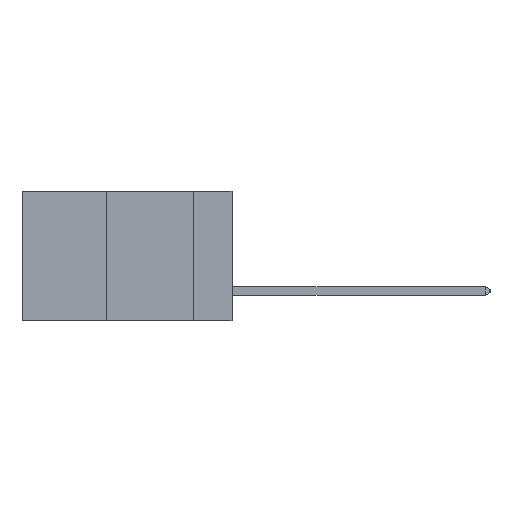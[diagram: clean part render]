
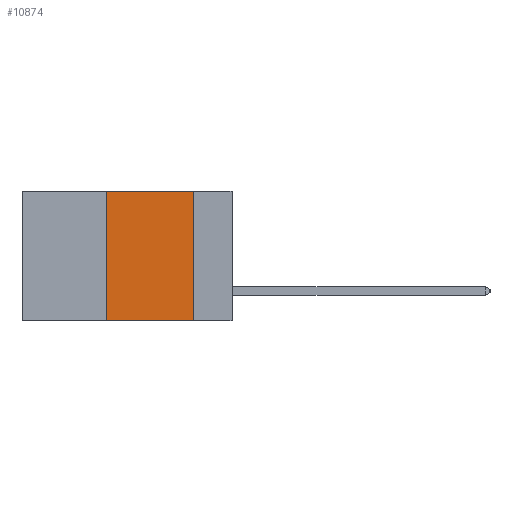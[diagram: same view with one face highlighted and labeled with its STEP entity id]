
A CAD part, left-side view. The second image highlights one B-rep face of the part: STEP entity #10874.
In plain terms, the highlighted planar face has unit normal (-1, 0, 0).
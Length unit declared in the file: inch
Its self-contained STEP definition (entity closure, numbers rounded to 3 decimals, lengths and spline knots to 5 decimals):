
#123 = CARTESIAN_POINT ( 'NONE',  ( 0., 0.6, -0.37 ) ) ;
#626 = ORIENTED_EDGE ( 'NONE', *, *, #4602, .F. ) ;
#1058 = DIRECTION ( 'NONE',  ( 0., 0., -1. ) ) ;
#1191 = AXIS2_PLACEMENT_3D ( 'NONE', #15369, #9246, #1058 ) ;
#1543 = DIRECTION ( 'NONE',  ( 0., -1., 0. ) ) ;
#2613 = CARTESIAN_POINT ( 'NONE',  ( 0., 0.11, 0. ) ) ;
#3537 = DIRECTION ( 'NONE',  ( 0., -1., 0. ) ) ;
#3974 = DIRECTION ( 'NONE',  ( 0., 0., -1. ) ) ;
#4198 = VECTOR ( 'NONE', #1543, 39.37008 ) ;
#4602 = EDGE_CURVE ( 'NONE', #4780, #7732, #5704, .T. ) ;
#4770 = EDGE_LOOP ( 'NONE', ( #626, #7957, #14985, #12144 ) ) ;
#4780 = VERTEX_POINT ( 'NONE', #15733 ) ;
#5704 = LINE ( 'NONE', #2613, #12165 ) ;
#6592 = VECTOR ( 'NONE', #9218, 39.37008 ) ;
#6851 = CARTESIAN_POINT ( 'NONE',  ( 0., 0.36, -0.37 ) ) ;
#7732 = VERTEX_POINT ( 'NONE', #9141 ) ;
#7957 = ORIENTED_EDGE ( 'NONE', *, *, #15161, .F. ) ;
#8431 = EDGE_CURVE ( 'NONE', #16558, #16662, #12989, .T. ) ;
#9141 = CARTESIAN_POINT ( 'NONE',  ( 0., 0.11, -0.37 ) ) ;
#9218 = DIRECTION ( 'NONE',  ( 0., 0., 1. ) ) ;
#9246 = DIRECTION ( 'NONE',  ( 1., 0., 0. ) ) ;
#9462 = VECTOR ( 'NONE', #3537, 39.37008 ) ;
#10874 = ADVANCED_FACE ( 'NONE', ( #12527 ), #12939, .F. ) ;
#12144 = ORIENTED_EDGE ( 'NONE', *, *, #16654, .T. ) ;
#12165 = VECTOR ( 'NONE', #3974, 39.37008 ) ;
#12527 = FACE_OUTER_BOUND ( 'NONE', #4770, .T. ) ;
#12710 = CARTESIAN_POINT ( 'NONE',  ( 0., 0.6, 0. ) ) ;
#12939 = PLANE ( 'NONE',  #1191 ) ;
#12989 = LINE ( 'NONE', #16570, #6592 ) ;
#13404 = CARTESIAN_POINT ( 'NONE',  ( 0., 0.36, 0. ) ) ;
#14847 = LINE ( 'NONE', #12710, #9462 ) ;
#14985 = ORIENTED_EDGE ( 'NONE', *, *, #8431, .F. ) ;
#15161 = EDGE_CURVE ( 'NONE', #16662, #4780, #14847, .T. ) ;
#15369 = CARTESIAN_POINT ( 'NONE',  ( 0., 0.6, 0. ) ) ;
#15733 = CARTESIAN_POINT ( 'NONE',  ( 0., 0.11, 0. ) ) ;
#16530 = LINE ( 'NONE', #123, #4198 ) ;
#16558 = VERTEX_POINT ( 'NONE', #6851 ) ;
#16570 = CARTESIAN_POINT ( 'NONE',  ( 0., 0.36, 0. ) ) ;
#16654 = EDGE_CURVE ( 'NONE', #16558, #7732, #16530, .T. ) ;
#16662 = VERTEX_POINT ( 'NONE', #13404 ) ;
